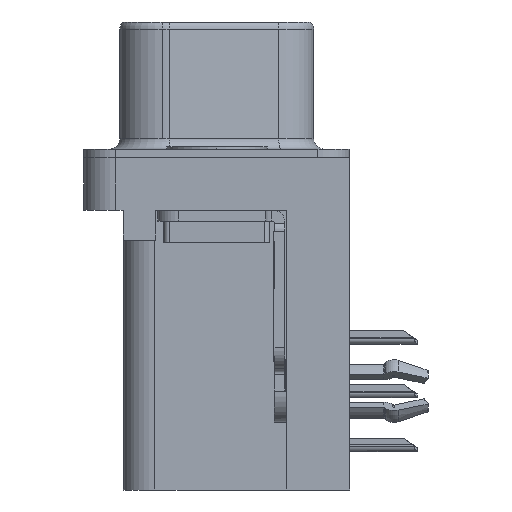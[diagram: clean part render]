
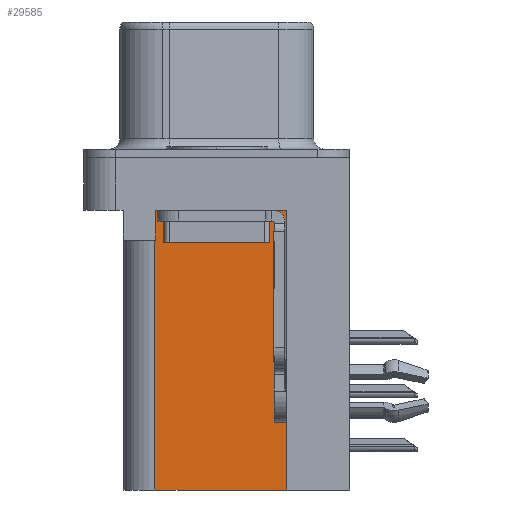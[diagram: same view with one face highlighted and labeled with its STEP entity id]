
A CAD part, left-side view. The second image highlights one B-rep face of the part: STEP entity #29585.
In plain terms, the highlighted planar face has unit normal (-1, 0, 0).
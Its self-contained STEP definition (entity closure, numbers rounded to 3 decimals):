
#794 = CARTESIAN_POINT ( 'NONE',  ( 3.79, -3.295, -15.7 ) ) ;
#898 = CARTESIAN_POINT ( 'NONE',  ( 3.79, 2.895, -3.9 ) ) ;
#1016 = EDGE_CURVE ( 'NONE', #6573, #22339, #32544, .T. ) ;
#1080 = EDGE_CURVE ( 'NONE', #6573, #31094, #23034, .T. ) ;
#1220 = DIRECTION ( 'NONE',  ( 0., 0., -1. ) ) ;
#1847 = EDGE_CURVE ( 'NONE', #31094, #5422, #5697, .T. ) ;
#3012 = ORIENTED_EDGE ( 'NONE', *, *, #33623, .T. ) ;
#4649 = VECTOR ( 'NONE', #26076, 1000. ) ;
#5137 = VECTOR ( 'NONE', #9991, 1000. ) ;
#5422 = VERTEX_POINT ( 'NONE', #9921 ) ;
#5697 = LINE ( 'NONE', #18823, #26524 ) ;
#6573 = VERTEX_POINT ( 'NONE', #23126 ) ;
#6863 = ORIENTED_EDGE ( 'NONE', *, *, #1847, .F. ) ;
#9333 = FACE_OUTER_BOUND ( 'NONE', #31835, .T. ) ;
#9921 = CARTESIAN_POINT ( 'NONE',  ( 3.79, 2.925, -3.9 ) ) ;
#9991 = DIRECTION ( 'NONE',  ( 0., 1., 0. ) ) ;
#10702 = EDGE_CURVE ( 'NONE', #17037, #34918, #14419, .T. ) ;
#12911 = CARTESIAN_POINT ( 'NONE',  ( 3.79, -3.295, -2.5 ) ) ;
#13080 = LINE ( 'NONE', #23185, #25579 ) ;
#14419 = LINE ( 'NONE', #898, #30129 ) ;
#14637 = DIRECTION ( 'NONE',  ( 0., 1., 0. ) ) ;
#15167 = PLANE ( 'NONE',  #26143 ) ;
#15974 = VECTOR ( 'NONE', #14637, 1000. ) ;
#16920 = ORIENTED_EDGE ( 'NONE', *, *, #10702, .T. ) ;
#17037 = VERTEX_POINT ( 'NONE', #26913 ) ;
#17350 = CARTESIAN_POINT ( 'NONE',  ( 3.79, 2.925, -15.7 ) ) ;
#17760 = DIRECTION ( 'NONE',  ( 1., 0., 0. ) ) ;
#17954 = DIRECTION ( 'NONE',  ( 0., 1., 0. ) ) ;
#18734 = CARTESIAN_POINT ( 'NONE',  ( 3.79, 2.895, -3.9 ) ) ;
#18823 = CARTESIAN_POINT ( 'NONE',  ( 3.79, 2.925, -15.7 ) ) ;
#18880 = LINE ( 'NONE', #26090, #5137 ) ;
#20139 = DIRECTION ( 'NONE',  ( 0., 0., -1. ) ) ;
#22339 = VERTEX_POINT ( 'NONE', #12911 ) ;
#23034 = LINE ( 'NONE', #794, #15974 ) ;
#23126 = CARTESIAN_POINT ( 'NONE',  ( 3.79, -3.295, -15.7 ) ) ;
#23185 = CARTESIAN_POINT ( 'NONE',  ( 3.79, 0., -3.9 ) ) ;
#24627 = EDGE_CURVE ( 'NONE', #34918, #5422, #13080, .T. ) ;
#24940 = CARTESIAN_POINT ( 'NONE',  ( 3.79, -3.295, -15.7 ) ) ;
#25579 = VECTOR ( 'NONE', #17954, 1000. ) ;
#26076 = DIRECTION ( 'NONE',  ( 0., 0., 1. ) ) ;
#26090 = CARTESIAN_POINT ( 'NONE',  ( 3.79, -3.295, -2.5 ) ) ;
#26143 = AXIS2_PLACEMENT_3D ( 'NONE', #30995, #17760, #1220 ) ;
#26524 = VECTOR ( 'NONE', #29061, 1000. ) ;
#26566 = ORIENTED_EDGE ( 'NONE', *, *, #1016, .T. ) ;
#26913 = CARTESIAN_POINT ( 'NONE',  ( 3.79, 2.895, -2.5 ) ) ;
#29061 = DIRECTION ( 'NONE',  ( 0., 0., 1. ) ) ;
#29585 = ADVANCED_FACE ( 'NONE', ( #9333 ), #15167, .F. ) ;
#30129 = VECTOR ( 'NONE', #20139, 1000. ) ;
#30995 = CARTESIAN_POINT ( 'NONE',  ( 3.79, -3.295, -15.7 ) ) ;
#31094 = VERTEX_POINT ( 'NONE', #17350 ) ;
#31835 = EDGE_LOOP ( 'NONE', ( #3012, #16920, #34172, #6863, #34592, #26566 ) ) ;
#32544 = LINE ( 'NONE', #24940, #4649 ) ;
#33623 = EDGE_CURVE ( 'NONE', #22339, #17037, #18880, .T. ) ;
#34172 = ORIENTED_EDGE ( 'NONE', *, *, #24627, .T. ) ;
#34592 = ORIENTED_EDGE ( 'NONE', *, *, #1080, .F. ) ;
#34918 = VERTEX_POINT ( 'NONE', #18734 ) ;
